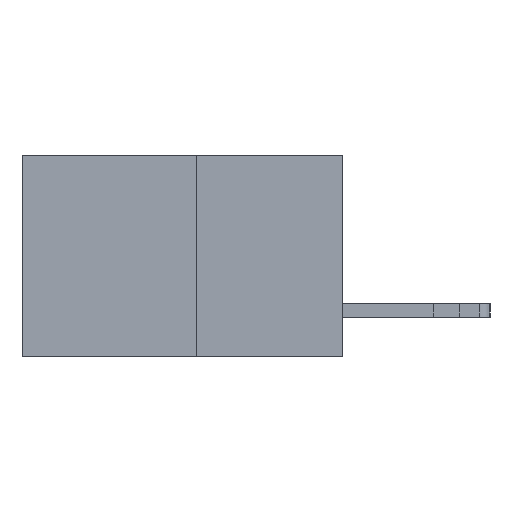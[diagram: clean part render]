
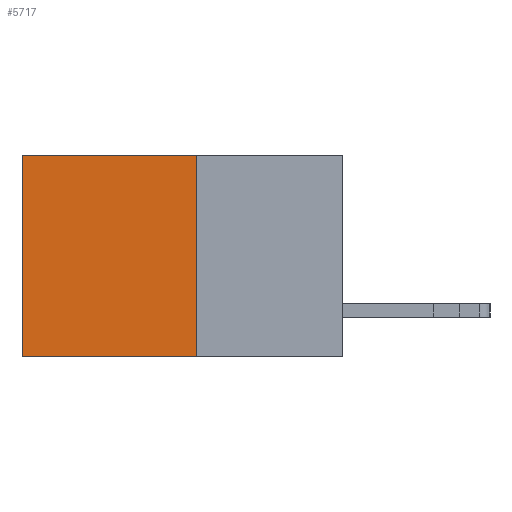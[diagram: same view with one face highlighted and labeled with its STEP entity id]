
A CAD part, left-side view. The second image highlights one B-rep face of the part: STEP entity #5717.
In plain terms, the highlighted planar face has unit normal (-1, 0, 0).
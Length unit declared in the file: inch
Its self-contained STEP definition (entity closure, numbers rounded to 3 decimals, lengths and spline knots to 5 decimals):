
#897 = ORIENTED_EDGE ( 'NONE', *, *, #2278, .T. ) ;
#1646 = LINE ( 'NONE', #4694, #8347 ) ;
#1938 = CARTESIAN_POINT ( 'NONE',  ( 0.277, 0.59, 0. ) ) ;
#2278 = EDGE_CURVE ( 'NONE', #11550, #13971, #3208, .T. ) ;
#2780 = VECTOR ( 'NONE', #5692, 39.37008 ) ;
#2862 = LINE ( 'NONE', #12042, #12856 ) ;
#2895 = VERTEX_POINT ( 'NONE', #8847 ) ;
#3148 = FACE_OUTER_BOUND ( 'NONE', #4220, .T. ) ;
#3208 = LINE ( 'NONE', #14753, #2780 ) ;
#4036 = DIRECTION ( 'NONE',  ( 0., 0., -1. ) ) ;
#4099 = DIRECTION ( 'NONE',  ( 1., 0., 0. ) ) ;
#4143 = CARTESIAN_POINT ( 'NONE',  ( 0.277, 0.27, -0.37 ) ) ;
#4215 = PLANE ( 'NONE',  #10118 ) ;
#4220 = EDGE_LOOP ( 'NONE', ( #897, #6692, #16464, #11699 ) ) ;
#4537 = DIRECTION ( 'NONE',  ( 0., 1., 0. ) ) ;
#4694 = CARTESIAN_POINT ( 'NONE',  ( 0.277, 0.27, 0. ) ) ;
#4701 = EDGE_CURVE ( 'NONE', #9655, #11550, #1646, .T. ) ;
#4821 = DIRECTION ( 'NONE',  ( 0., 1., 0. ) ) ;
#5224 = CARTESIAN_POINT ( 'NONE',  ( 0.277, 0.27, -0.37 ) ) ;
#5660 = EDGE_CURVE ( 'NONE', #2895, #13971, #14262, .T. ) ;
#5692 = DIRECTION ( 'NONE',  ( 0., 0., -1. ) ) ;
#5717 = ADVANCED_FACE ( 'NONE', ( #3148 ), #4215, .F. ) ;
#6692 = ORIENTED_EDGE ( 'NONE', *, *, #5660, .F. ) ;
#7527 = CARTESIAN_POINT ( 'NONE',  ( 0.277, 0.27, 0. ) ) ;
#7634 = EDGE_CURVE ( 'NONE', #9655, #2895, #2862, .T. ) ;
#8347 = VECTOR ( 'NONE', #4537, 39.37008 ) ;
#8847 = CARTESIAN_POINT ( 'NONE',  ( 0.277, 0.27, -0.37 ) ) ;
#9655 = VERTEX_POINT ( 'NONE', #7527 ) ;
#10118 = AXIS2_PLACEMENT_3D ( 'NONE', #4143, #4099, #4036 ) ;
#11550 = VERTEX_POINT ( 'NONE', #1938 ) ;
#11699 = ORIENTED_EDGE ( 'NONE', *, *, #4701, .T. ) ;
#11818 = DIRECTION ( 'NONE',  ( 0., 0., -1. ) ) ;
#12042 = CARTESIAN_POINT ( 'NONE',  ( 0.277, 0.27, -0.37 ) ) ;
#12594 = CARTESIAN_POINT ( 'NONE',  ( 0.277, 0.59, -0.37 ) ) ;
#12856 = VECTOR ( 'NONE', #11818, 39.37008 ) ;
#13862 = VECTOR ( 'NONE', #4821, 39.37008 ) ;
#13971 = VERTEX_POINT ( 'NONE', #12594 ) ;
#14262 = LINE ( 'NONE', #5224, #13862 ) ;
#14753 = CARTESIAN_POINT ( 'NONE',  ( 0.277, 0.59, -0.37 ) ) ;
#16464 = ORIENTED_EDGE ( 'NONE', *, *, #7634, .F. ) ;
